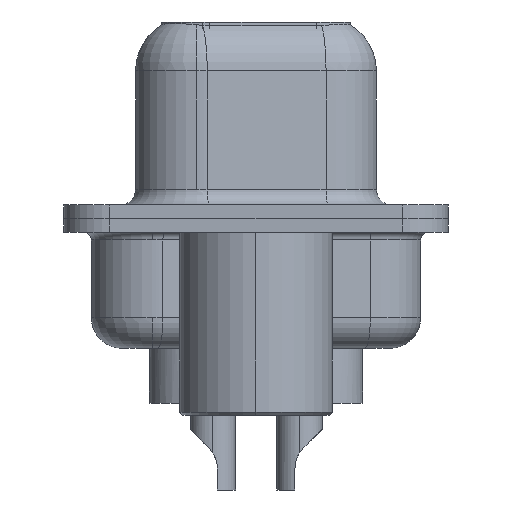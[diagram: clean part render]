
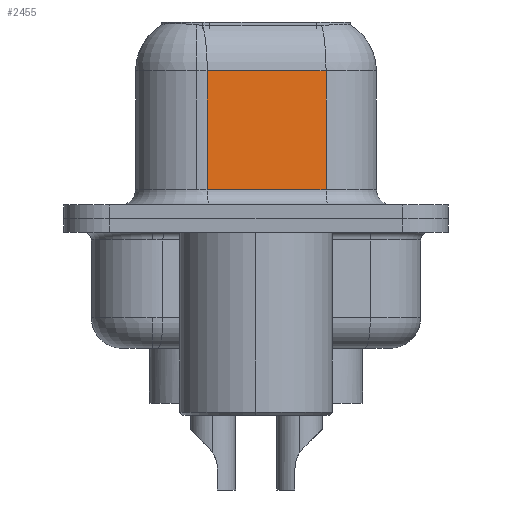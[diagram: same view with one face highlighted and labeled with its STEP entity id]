
A CAD part, left-side view. The second image highlights one B-rep face of the part: STEP entity #2455.
In plain terms, the highlighted planar face has unit normal (-0.985, -0.174, 0).
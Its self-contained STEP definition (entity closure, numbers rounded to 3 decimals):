
#288 = EDGE_CURVE ( 'NONE', #10784, #2486, #950, .T. ) ;
#950 = LINE ( 'NONE', #14383, #8583 ) ;
#1158 = ORIENTED_EDGE ( 'NONE', *, *, #288, .T. ) ;
#1660 = EDGE_CURVE ( 'NONE', #5796, #14531, #21700, .T. ) ;
#2455 = ADVANCED_FACE ( 'NONE', ( #17688 ), #21266, .F. ) ;
#2486 = VERTEX_POINT ( 'NONE', #6387 ) ;
#4828 = VECTOR ( 'NONE', #20269, 1000. ) ;
#4937 = CARTESIAN_POINT ( 'NONE',  ( 5.053, -2.297, 6.6 ) ) ;
#5796 = VERTEX_POINT ( 'NONE', #6087 ) ;
#5907 = EDGE_CURVE ( 'NONE', #10784, #14531, #10254, .T. ) ;
#6087 = CARTESIAN_POINT ( 'NONE',  ( 4.365, 1.603, 0.95 ) ) ;
#6387 = CARTESIAN_POINT ( 'NONE',  ( 4.365, 1.603, 4.85 ) ) ;
#7439 = DIRECTION ( 'NONE',  ( 0.985, 0.174, 0. ) ) ;
#8583 = VECTOR ( 'NONE', #13041, 1000. ) ;
#10254 = LINE ( 'NONE', #4937, #4828 ) ;
#10698 = VECTOR ( 'NONE', #14148, 1000. ) ;
#10784 = VERTEX_POINT ( 'NONE', #16151 ) ;
#12048 = EDGE_CURVE ( 'NONE', #2486, #5796, #20593, .T. ) ;
#12428 = ORIENTED_EDGE ( 'NONE', *, *, #5907, .F. ) ;
#13041 = DIRECTION ( 'NONE',  ( -0.174, 0.985, 0. ) ) ;
#13095 = CARTESIAN_POINT ( 'NONE',  ( 5.053, -2.297, 0.95 ) ) ;
#13125 = CARTESIAN_POINT ( 'NONE',  ( 5.053, -2.297, 0.95 ) ) ;
#13202 = DIRECTION ( 'NONE',  ( 0.174, -0.985, 0. ) ) ;
#14148 = DIRECTION ( 'NONE',  ( 0., 0., -1. ) ) ;
#14383 = CARTESIAN_POINT ( 'NONE',  ( 5.053, -2.297, 4.85 ) ) ;
#14531 = VERTEX_POINT ( 'NONE', #13125 ) ;
#16151 = CARTESIAN_POINT ( 'NONE',  ( 5.053, -2.297, 4.85 ) ) ;
#17377 = CARTESIAN_POINT ( 'NONE',  ( 4.365, 1.603, 6.6 ) ) ;
#17688 = FACE_OUTER_BOUND ( 'NONE', #19640, .T. ) ;
#17903 = CARTESIAN_POINT ( 'NONE',  ( 5.053, -2.297, 6.6 ) ) ;
#19640 = EDGE_LOOP ( 'NONE', ( #12428, #1158, #21511, #21456 ) ) ;
#19659 = VECTOR ( 'NONE', #13202, 1000. ) ;
#20269 = DIRECTION ( 'NONE',  ( 0., 0., -1. ) ) ;
#20593 = LINE ( 'NONE', #17377, #10698 ) ;
#21039 = DIRECTION ( 'NONE',  ( -0.174, 0.985, 0. ) ) ;
#21266 = PLANE ( 'NONE',  #21895 ) ;
#21456 = ORIENTED_EDGE ( 'NONE', *, *, #1660, .T. ) ;
#21511 = ORIENTED_EDGE ( 'NONE', *, *, #12048, .T. ) ;
#21700 = LINE ( 'NONE', #13095, #19659 ) ;
#21895 = AXIS2_PLACEMENT_3D ( 'NONE', #17903, #7439, #21039 ) ;
